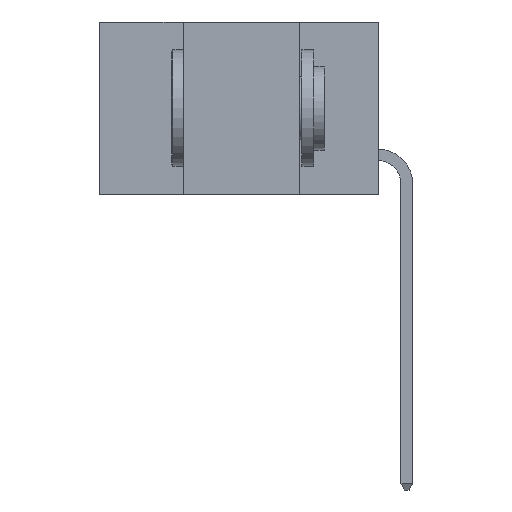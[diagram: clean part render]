
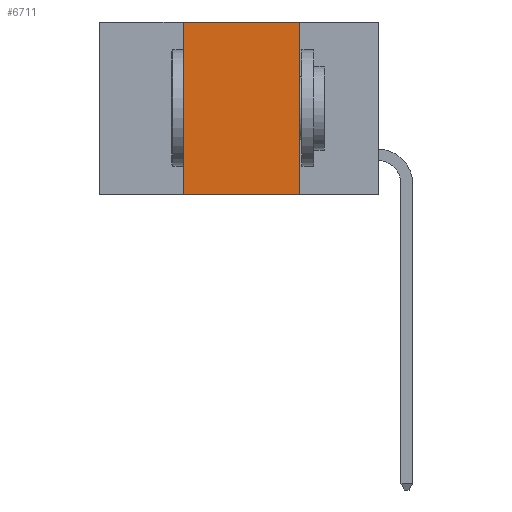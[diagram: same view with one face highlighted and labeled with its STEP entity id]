
A CAD part, left-side view. The second image highlights one B-rep face of the part: STEP entity #6711.
In plain terms, the highlighted planar face has unit normal (-1, 0, 0).
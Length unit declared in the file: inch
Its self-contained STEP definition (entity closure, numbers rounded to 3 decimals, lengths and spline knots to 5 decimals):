
#338 = ORIENTED_EDGE ( 'NONE', *, *, #5284, .T. ) ;
#1603 = CARTESIAN_POINT ( 'NONE',  ( 0., 0.6, 0. ) ) ;
#3168 = CARTESIAN_POINT ( 'NONE',  ( 0., 0.6, -0.37 ) ) ;
#3244 = CARTESIAN_POINT ( 'NONE',  ( 0., 0.17, -0.37 ) ) ;
#5284 = EDGE_CURVE ( 'NONE', #19857, #13143, #13695, .T. ) ;
#6574 = DIRECTION ( 'NONE',  ( 0., -1., 0. ) ) ;
#6711 = ADVANCED_FACE ( 'NONE', ( #10775 ), #9786, .F. ) ;
#7112 = EDGE_CURVE ( 'NONE', #19857, #13745, #16795, .T. ) ;
#7917 = ORIENTED_EDGE ( 'NONE', *, *, #7112, .F. ) ;
#8027 = EDGE_CURVE ( 'NONE', #16601, #13143, #21067, .T. ) ;
#8732 = DIRECTION ( 'NONE',  ( 0., 0., -1. ) ) ;
#9385 = DIRECTION ( 'NONE',  ( 1., 0., 0. ) ) ;
#9620 = CARTESIAN_POINT ( 'NONE',  ( 0., 0.6, 0. ) ) ;
#9786 = PLANE ( 'NONE',  #14736 ) ;
#10775 = FACE_OUTER_BOUND ( 'NONE', #13927, .T. ) ;
#10957 = VECTOR ( 'NONE', #17743, 39.37008 ) ;
#11310 = EDGE_CURVE ( 'NONE', #13745, #16601, #16220, .T. ) ;
#13143 = VERTEX_POINT ( 'NONE', #13950 ) ;
#13695 = LINE ( 'NONE', #3168, #17782 ) ;
#13745 = VERTEX_POINT ( 'NONE', #25705 ) ;
#13927 = EDGE_LOOP ( 'NONE', ( #15016, #15366, #7917, #338 ) ) ;
#13950 = CARTESIAN_POINT ( 'NONE',  ( 0., 0.17, -0.37 ) ) ;
#14736 = AXIS2_PLACEMENT_3D ( 'NONE', #9620, #9385, #8732 ) ;
#15016 = ORIENTED_EDGE ( 'NONE', *, *, #8027, .F. ) ;
#15366 = ORIENTED_EDGE ( 'NONE', *, *, #11310, .F. ) ;
#15619 = CARTESIAN_POINT ( 'NONE',  ( 0., 0.42, -0.37 ) ) ;
#16220 = LINE ( 'NONE', #1603, #20929 ) ;
#16601 = VERTEX_POINT ( 'NONE', #25727 ) ;
#16795 = LINE ( 'NONE', #16869, #17417 ) ;
#16869 = CARTESIAN_POINT ( 'NONE',  ( 0., 0.42, -0.37 ) ) ;
#16959 = DIRECTION ( 'NONE',  ( 0., 0., 1. ) ) ;
#17417 = VECTOR ( 'NONE', #16959, 39.37008 ) ;
#17743 = DIRECTION ( 'NONE',  ( 0., 0., -1. ) ) ;
#17782 = VECTOR ( 'NONE', #6574, 39.37008 ) ;
#19857 = VERTEX_POINT ( 'NONE', #15619 ) ;
#20929 = VECTOR ( 'NONE', #22086, 39.37008 ) ;
#21067 = LINE ( 'NONE', #3244, #10957 ) ;
#22086 = DIRECTION ( 'NONE',  ( 0., -1., 0. ) ) ;
#25705 = CARTESIAN_POINT ( 'NONE',  ( 0., 0.42, 0. ) ) ;
#25727 = CARTESIAN_POINT ( 'NONE',  ( 0., 0.17, 0. ) ) ;
